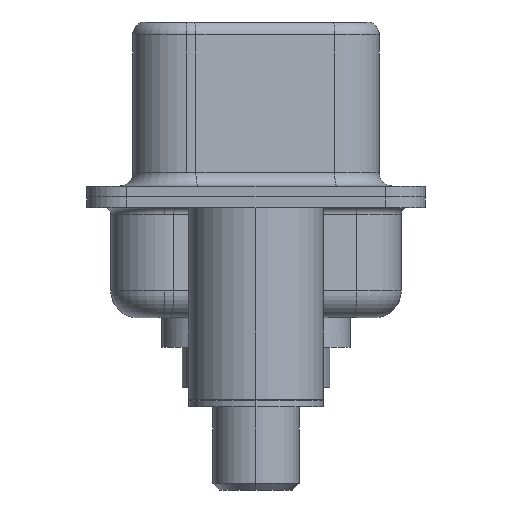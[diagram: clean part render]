
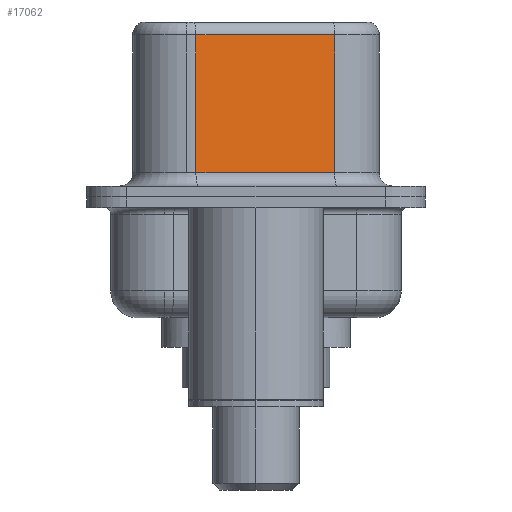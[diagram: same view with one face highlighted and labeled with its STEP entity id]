
A CAD part, left-side view. The second image highlights one B-rep face of the part: STEP entity #17062.
In plain terms, the highlighted planar face has unit normal (-0.985, -0.174, 0).
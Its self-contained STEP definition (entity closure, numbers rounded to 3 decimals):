
#161 = VECTOR ( 'NONE', #15616, 1000. ) ;
#971 = VERTEX_POINT ( 'NONE', #10881 ) ;
#1758 = CARTESIAN_POINT ( 'NONE',  ( 3.655, 2.233, 6.52 ) ) ;
#2077 = EDGE_CURVE ( 'NONE', #14430, #6422, #8360, .T. ) ;
#2152 = ORIENTED_EDGE ( 'NONE', *, *, #15850, .T. ) ;
#2214 = CARTESIAN_POINT ( 'NONE',  ( 3.655, 2.233, 0.9 ) ) ;
#3305 = DIRECTION ( 'NONE',  ( 0., 0., -1. ) ) ;
#3628 = CARTESIAN_POINT ( 'NONE',  ( 4.565, -2.927, 6.02 ) ) ;
#4243 = AXIS2_PLACEMENT_3D ( 'NONE', #8437, #5332, #16087 ) ;
#4356 = VECTOR ( 'NONE', #7273, 1000. ) ;
#4475 = VERTEX_POINT ( 'NONE', #2214 ) ;
#5172 = FACE_OUTER_BOUND ( 'NONE', #11268, .T. ) ;
#5332 = DIRECTION ( 'NONE',  ( 0.985, 0.174, 0. ) ) ;
#5349 = EDGE_CURVE ( 'NONE', #14430, #971, #13105, .T. ) ;
#6422 = VERTEX_POINT ( 'NONE', #13013 ) ;
#7273 = DIRECTION ( 'NONE',  ( -0.174, 0.985, 0. ) ) ;
#7871 = CARTESIAN_POINT ( 'NONE',  ( 4.565, -2.927, 6.52 ) ) ;
#8360 = LINE ( 'NONE', #7871, #161 ) ;
#8437 = CARTESIAN_POINT ( 'NONE',  ( 4.565, -2.927, 6.52 ) ) ;
#8924 = ORIENTED_EDGE ( 'NONE', *, *, #2077, .F. ) ;
#9442 = DIRECTION ( 'NONE',  ( 0.174, -0.985, 0. ) ) ;
#9712 = ORIENTED_EDGE ( 'NONE', *, *, #5349, .T. ) ;
#9716 = ORIENTED_EDGE ( 'NONE', *, *, #10182, .T. ) ;
#9867 = VECTOR ( 'NONE', #9442, 1000. ) ;
#10017 = VECTOR ( 'NONE', #3305, 1000. ) ;
#10182 = EDGE_CURVE ( 'NONE', #971, #4475, #14579, .T. ) ;
#10881 = CARTESIAN_POINT ( 'NONE',  ( 3.655, 2.233, 6.02 ) ) ;
#11268 = EDGE_LOOP ( 'NONE', ( #8924, #9712, #9716, #2152 ) ) ;
#11556 = PLANE ( 'NONE',  #4243 ) ;
#13013 = CARTESIAN_POINT ( 'NONE',  ( 4.565, -2.927, 0.9 ) ) ;
#13105 = LINE ( 'NONE', #19451, #4356 ) ;
#14430 = VERTEX_POINT ( 'NONE', #3628 ) ;
#14579 = LINE ( 'NONE', #1758, #10017 ) ;
#15616 = DIRECTION ( 'NONE',  ( 0., 0., -1. ) ) ;
#15850 = EDGE_CURVE ( 'NONE', #4475, #6422, #17928, .T. ) ;
#16087 = DIRECTION ( 'NONE',  ( -0.174, 0.985, 0. ) ) ;
#17062 = ADVANCED_FACE ( 'NONE', ( #5172 ), #11556, .F. ) ;
#17928 = LINE ( 'NONE', #18531, #9867 ) ;
#18531 = CARTESIAN_POINT ( 'NONE',  ( 4.565, -2.927, 0.9 ) ) ;
#19451 = CARTESIAN_POINT ( 'NONE',  ( 4.565, -2.927, 6.02 ) ) ;
